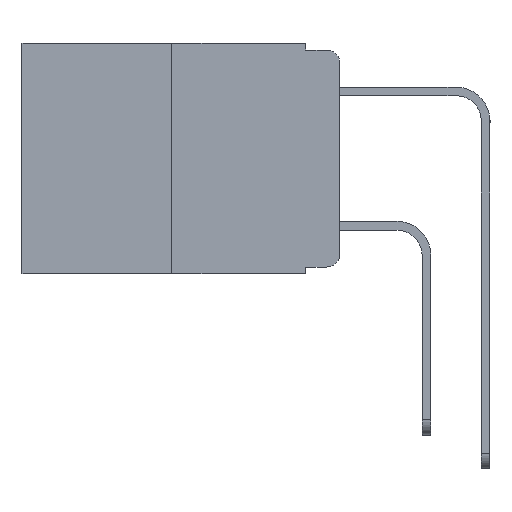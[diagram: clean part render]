
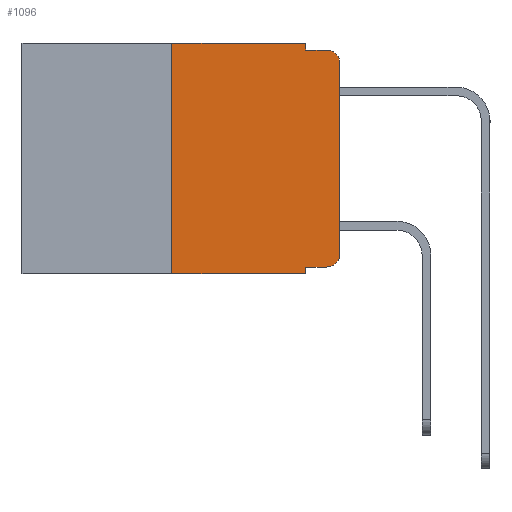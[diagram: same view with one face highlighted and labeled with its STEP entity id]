
A CAD part, left-side view. The second image highlights one B-rep face of the part: STEP entity #1096.
In plain terms, the highlighted planar face has unit normal (-1, 0, 0).
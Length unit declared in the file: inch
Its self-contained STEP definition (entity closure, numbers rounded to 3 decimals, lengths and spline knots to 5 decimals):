
#479 = ORIENTED_EDGE ( 'NONE', *, *, #7262, .T. ) ;
#684 = CARTESIAN_POINT ( 'NONE',  ( 0., 0.473, 0. ) ) ;
#760 = CARTESIAN_POINT ( 'NONE',  ( 0., 0.051, -0.01 ) ) ;
#762 = CARTESIAN_POINT ( 'NONE',  ( 0., 0.051, -0.333 ) ) ;
#879 = LINE ( 'NONE', #2776, #9032 ) ;
#1022 = VERTEX_POINT ( 'NONE', #5119 ) ;
#1096 = ADVANCED_FACE ( 'NONE', ( #12318 ), #5509, .F. ) ;
#1254 = VECTOR ( 'NONE', #5653, 39.37008 ) ;
#1374 = VECTOR ( 'NONE', #6582, 39.37008 ) ;
#1529 = VERTEX_POINT ( 'NONE', #6660 ) ;
#1557 = VECTOR ( 'NONE', #13346, 39.37008 ) ;
#1591 = LINE ( 'NONE', #5692, #1254 ) ;
#1639 = DIRECTION ( 'NONE',  ( 0., 0., -1. ) ) ;
#1780 = EDGE_CURVE ( 'NONE', #12583, #8578, #4355, .T. ) ;
#1841 = EDGE_CURVE ( 'NONE', #11239, #1022, #879, .T. ) ;
#2117 = VECTOR ( 'NONE', #11316, 39.37008 ) ;
#2294 = EDGE_CURVE ( 'NONE', #1529, #13540, #3675, .T. ) ;
#2311 = ORIENTED_EDGE ( 'NONE', *, *, #4692, .F. ) ;
#2458 = LINE ( 'NONE', #684, #2117 ) ;
#2584 = CARTESIAN_POINT ( 'NONE',  ( 0., 0.051, -0.343 ) ) ;
#2776 = CARTESIAN_POINT ( 'NONE',  ( 0., 0.051, 0. ) ) ;
#3629 = CARTESIAN_POINT ( 'NONE',  ( 0., 0., -0.313 ) ) ;
#3675 = CIRCLE ( 'NONE', #4248, 0.02 ) ;
#3930 = EDGE_LOOP ( 'NONE', ( #479, #8618, #2311, #12546, #11914, #6267, #4277, #12401, #10501, #12559 ) ) ;
#4174 = LINE ( 'NONE', #7670, #1374 ) ;
#4215 = VERTEX_POINT ( 'NONE', #762 ) ;
#4248 = AXIS2_PLACEMENT_3D ( 'NONE', #11784, #9489, #6488 ) ;
#4277 = ORIENTED_EDGE ( 'NONE', *, *, #13416, .T. ) ;
#4348 = LINE ( 'NONE', #8949, #6844 ) ;
#4355 = LINE ( 'NONE', #11198, #1557 ) ;
#4547 = LINE ( 'NONE', #8174, #12626 ) ;
#4692 = EDGE_CURVE ( 'NONE', #1022, #13540, #10765, .T. ) ;
#4725 = DIRECTION ( 'NONE',  ( 0., -1., 0. ) ) ;
#4817 = CARTESIAN_POINT ( 'NONE',  ( 0., 0.02, -0.333 ) ) ;
#4941 = CARTESIAN_POINT ( 'NONE',  ( 0., 0.051, 0. ) ) ;
#5119 = CARTESIAN_POINT ( 'NONE',  ( 0., 0.051, -0.01 ) ) ;
#5424 = CARTESIAN_POINT ( 'NONE',  ( 0., 0.473, 0. ) ) ;
#5509 = PLANE ( 'NONE',  #6299 ) ;
#5653 = DIRECTION ( 'NONE',  ( 0., 0., -1. ) ) ;
#5692 = CARTESIAN_POINT ( 'NONE',  ( 0., 0.051, 0. ) ) ;
#5883 = DIRECTION ( 'NONE',  ( 1., 0., 0. ) ) ;
#5911 = DIRECTION ( 'NONE',  ( 0., 0., -1. ) ) ;
#5934 = DIRECTION ( 'NONE',  ( -1., 0., 0. ) ) ;
#6267 = ORIENTED_EDGE ( 'NONE', *, *, #1780, .F. ) ;
#6299 = AXIS2_PLACEMENT_3D ( 'NONE', #5424, #5883, #5911 ) ;
#6488 = DIRECTION ( 'NONE',  ( 0., 0., -1. ) ) ;
#6529 = EDGE_CURVE ( 'NONE', #4215, #11044, #1591, .T. ) ;
#6582 = DIRECTION ( 'NONE',  ( 0., -1., 0. ) ) ;
#6660 = CARTESIAN_POINT ( 'NONE',  ( 0., 0., -0.03 ) ) ;
#6844 = VECTOR ( 'NONE', #4725, 39.37008 ) ;
#7223 = DIRECTION ( 'NONE',  ( 0., -1., 0. ) ) ;
#7261 = CARTESIAN_POINT ( 'NONE',  ( 0., 0.25, -0.343 ) ) ;
#7262 = EDGE_CURVE ( 'NONE', #12899, #1529, #4547, .T. ) ;
#7670 = CARTESIAN_POINT ( 'NONE',  ( 0., 0.473, -0.343 ) ) ;
#7736 = CIRCLE ( 'NONE', #13144, 0.02 ) ;
#7988 = EDGE_CURVE ( 'NONE', #4215, #10081, #4348, .T. ) ;
#8174 = CARTESIAN_POINT ( 'NONE',  ( 0., 0., 0. ) ) ;
#8578 = VERTEX_POINT ( 'NONE', #12014 ) ;
#8618 = ORIENTED_EDGE ( 'NONE', *, *, #2294, .T. ) ;
#8949 = CARTESIAN_POINT ( 'NONE',  ( 0., 0.051, -0.333 ) ) ;
#9032 = VECTOR ( 'NONE', #1639, 39.37008 ) ;
#9468 = EDGE_CURVE ( 'NONE', #8578, #11239, #2458, .T. ) ;
#9489 = DIRECTION ( 'NONE',  ( -1., 0., 0. ) ) ;
#10081 = VERTEX_POINT ( 'NONE', #4817 ) ;
#10501 = ORIENTED_EDGE ( 'NONE', *, *, #7988, .T. ) ;
#10765 = LINE ( 'NONE', #760, #13512 ) ;
#10808 = EDGE_CURVE ( 'NONE', #10081, #12899, #7736, .T. ) ;
#11044 = VERTEX_POINT ( 'NONE', #2584 ) ;
#11198 = CARTESIAN_POINT ( 'NONE',  ( 0., 0.25, 0. ) ) ;
#11239 = VERTEX_POINT ( 'NONE', #4941 ) ;
#11316 = DIRECTION ( 'NONE',  ( 0., -1., 0. ) ) ;
#11784 = CARTESIAN_POINT ( 'NONE',  ( 0., 0.02, -0.03 ) ) ;
#11914 = ORIENTED_EDGE ( 'NONE', *, *, #9468, .F. ) ;
#12014 = CARTESIAN_POINT ( 'NONE',  ( 0., 0.25, 0. ) ) ;
#12092 = CARTESIAN_POINT ( 'NONE',  ( 0., 0.02, -0.01 ) ) ;
#12265 = CARTESIAN_POINT ( 'NONE',  ( 0., 0.02, -0.313 ) ) ;
#12318 = FACE_OUTER_BOUND ( 'NONE', #3930, .T. ) ;
#12380 = DIRECTION ( 'NONE',  ( 0., 0., 1. ) ) ;
#12401 = ORIENTED_EDGE ( 'NONE', *, *, #6529, .F. ) ;
#12546 = ORIENTED_EDGE ( 'NONE', *, *, #1841, .F. ) ;
#12559 = ORIENTED_EDGE ( 'NONE', *, *, #10808, .T. ) ;
#12583 = VERTEX_POINT ( 'NONE', #7261 ) ;
#12626 = VECTOR ( 'NONE', #12380, 39.37008 ) ;
#12899 = VERTEX_POINT ( 'NONE', #3629 ) ;
#13144 = AXIS2_PLACEMENT_3D ( 'NONE', #12265, #5934, #13297 ) ;
#13297 = DIRECTION ( 'NONE',  ( 0., 0., -1. ) ) ;
#13346 = DIRECTION ( 'NONE',  ( 0., 0., 1. ) ) ;
#13416 = EDGE_CURVE ( 'NONE', #12583, #11044, #4174, .T. ) ;
#13512 = VECTOR ( 'NONE', #7223, 39.37008 ) ;
#13540 = VERTEX_POINT ( 'NONE', #12092 ) ;
